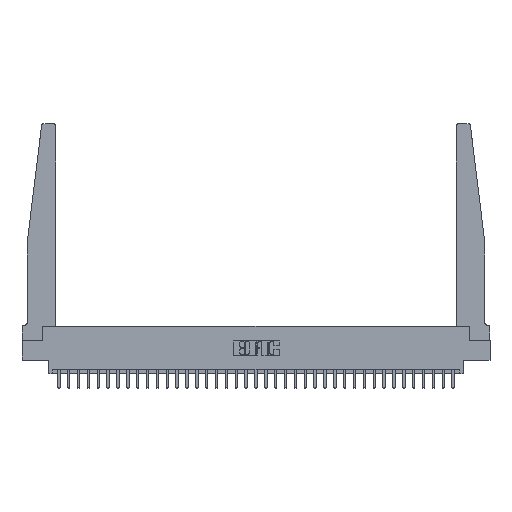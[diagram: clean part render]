
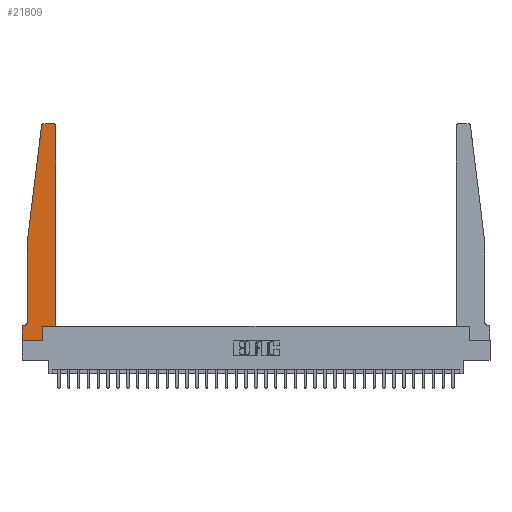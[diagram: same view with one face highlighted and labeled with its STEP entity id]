
A CAD part, top view. The second image highlights one B-rep face of the part: STEP entity #21809.
In plain terms, the highlighted planar face has unit normal (0, 0, 1).
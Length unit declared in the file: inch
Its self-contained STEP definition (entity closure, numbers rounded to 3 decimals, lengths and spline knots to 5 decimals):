
#943 = CARTESIAN_POINT ( 'NONE',  ( 0., 0., 0.37 ) ) ;
#962 = VERTEX_POINT ( 'NONE', #7965 ) ;
#1593 = CIRCLE ( 'NONE', #13711, 0.03 ) ;
#1871 = AXIS2_PLACEMENT_3D ( 'NONE', #12063, #29460, #30108 ) ;
#1919 = VECTOR ( 'NONE', #22863, 39.37008 ) ;
#2010 = CARTESIAN_POINT ( 'NONE',  ( 0.425, 0.18, 0.37 ) ) ;
#2086 = CARTESIAN_POINT ( 'NONE',  ( 0.065, 1.25, 0.37 ) ) ;
#2174 = DIRECTION ( 'NONE',  ( 0., 0., 1. ) ) ;
#2515 = CARTESIAN_POINT ( 'NONE',  ( 0., 0., 0.37 ) ) ;
#2569 = LINE ( 'NONE', #2086, #29321 ) ;
#2883 = CARTESIAN_POINT ( 'NONE',  ( 0.27653, 2.75, 0.37 ) ) ;
#3471 = CARTESIAN_POINT ( 'NONE',  ( 0.425, 0.18, 0.37 ) ) ;
#3569 = VERTEX_POINT ( 'NONE', #27847 ) ;
#3655 = CARTESIAN_POINT ( 'NONE',  ( 0.065, 0.1875, 0.37 ) ) ;
#4301 = ORIENTED_EDGE ( 'NONE', *, *, #28901, .T. ) ;
#5416 = ORIENTED_EDGE ( 'NONE', *, *, #29785, .T. ) ;
#5921 = CIRCLE ( 'NONE', #12198, 0.03 ) ;
#6221 = VECTOR ( 'NONE', #16796, 39.37008 ) ;
#6303 = EDGE_CURVE ( 'NONE', #18029, #8403, #32138, .T. ) ;
#6345 = ORIENTED_EDGE ( 'NONE', *, *, #8259, .T. ) ;
#6392 = VERTEX_POINT ( 'NONE', #14116 ) ;
#6654 = ORIENTED_EDGE ( 'NONE', *, *, #11583, .T. ) ;
#6799 = CARTESIAN_POINT ( 'NONE',  ( 0.25, 2.75, 0.37 ) ) ;
#7400 = ORIENTED_EDGE ( 'NONE', *, *, #25180, .T. ) ;
#7965 = CARTESIAN_POINT ( 'NONE',  ( 0.065, 1.25, 0.37 ) ) ;
#7969 = EDGE_CURVE ( 'NONE', #3569, #21873, #12035, .T. ) ;
#8115 = VERTEX_POINT ( 'NONE', #21014 ) ;
#8259 = EDGE_CURVE ( 'NONE', #16986, #6392, #22028, .T. ) ;
#8403 = VERTEX_POINT ( 'NONE', #2010 ) ;
#8548 = DIRECTION ( 'NONE',  ( 0., -1., 0. ) ) ;
#9052 = DIRECTION ( 'NONE',  ( 0., 0., -1. ) ) ;
#9510 = DIRECTION ( 'NONE',  ( 1., 0., 0. ) ) ;
#10059 = VECTOR ( 'NONE', #13225, 39.37008 ) ;
#10998 = DIRECTION ( 'NONE',  ( 0., 1., 0. ) ) ;
#11488 = CARTESIAN_POINT ( 'NONE',  ( 0., 0., 0.37 ) ) ;
#11583 = EDGE_CURVE ( 'NONE', #22275, #18432, #28152, .T. ) ;
#12035 = LINE ( 'NONE', #6799, #6221 ) ;
#12063 = CARTESIAN_POINT ( 'NONE',  ( 0., 0.1875, 0.37 ) ) ;
#12198 = AXIS2_PLACEMENT_3D ( 'NONE', #18623, #21079, #13717 ) ;
#12219 = CARTESIAN_POINT ( 'NONE',  ( 0.425, 2.72, 0.37 ) ) ;
#12319 = CARTESIAN_POINT ( 'NONE',  ( 0.395, 2.72, 0.37 ) ) ;
#13225 = DIRECTION ( 'NONE',  ( 1., 0., 0. ) ) ;
#13678 = EDGE_CURVE ( 'NONE', #27486, #962, #17900, .T. ) ;
#13711 = AXIS2_PLACEMENT_3D ( 'NONE', #12319, #2174, #17070 ) ;
#13717 = DIRECTION ( 'NONE',  ( 1., 0., 0. ) ) ;
#14116 = CARTESIAN_POINT ( 'NONE',  ( 0.015, 0.1875, 0.37 ) ) ;
#14307 = DIRECTION ( 'NONE',  ( -1., 0., 0. ) ) ;
#14493 = ORIENTED_EDGE ( 'NONE', *, *, #13678, .T. ) ;
#15130 = DIRECTION ( 'NONE',  ( -0.122, -0.992, 0. ) ) ;
#15173 = FACE_OUTER_BOUND ( 'NONE', #15773, .T. ) ;
#15477 = ORIENTED_EDGE ( 'NONE', *, *, #23230, .T. ) ;
#15773 = EDGE_LOOP ( 'NONE', ( #28804, #21388, #14493, #4301, #6345, #7400, #28339, #6654, #15477, #23433, #24573, #5416 ) ) ;
#15919 = LINE ( 'NONE', #3471, #27981 ) ;
#16796 = DIRECTION ( 'NONE',  ( -1., 0., 0. ) ) ;
#16986 = VERTEX_POINT ( 'NONE', #21519 ) ;
#17070 = DIRECTION ( 'NONE',  ( 1., 0., 0. ) ) ;
#17461 = PLANE ( 'NONE',  #1871 ) ;
#17900 = LINE ( 'NONE', #22816, #29016 ) ;
#18029 = VERTEX_POINT ( 'NONE', #22697 ) ;
#18432 = VERTEX_POINT ( 'NONE', #22808 ) ;
#18623 = CARTESIAN_POINT ( 'NONE',  ( 0.27653, 2.72, 0.37 ) ) ;
#19140 = EDGE_CURVE ( 'NONE', #21873, #27486, #5921, .T. ) ;
#19248 = VERTEX_POINT ( 'NONE', #12219 ) ;
#19409 = AXIS2_PLACEMENT_3D ( 'NONE', #26441, #9052, #14307 ) ;
#20860 = EDGE_CURVE ( 'NONE', #8403, #19248, #15919, .T. ) ;
#21014 = CARTESIAN_POINT ( 'NONE',  ( 0., 0.1875, 0.37 ) ) ;
#21079 = DIRECTION ( 'NONE',  ( 0., 0., 1. ) ) ;
#21388 = ORIENTED_EDGE ( 'NONE', *, *, #19140, .T. ) ;
#21519 = CARTESIAN_POINT ( 'NONE',  ( 0.065, 0.2375, 0.37 ) ) ;
#21809 = ADVANCED_FACE ( 'NONE', ( #15173 ), #17461, .T. ) ;
#21873 = VERTEX_POINT ( 'NONE', #2883 ) ;
#22028 = CIRCLE ( 'NONE', #19409, 0.05 ) ;
#22275 = VERTEX_POINT ( 'NONE', #2515 ) ;
#22387 = DIRECTION ( 'NONE',  ( 0., -1., 0. ) ) ;
#22697 = CARTESIAN_POINT ( 'NONE',  ( 0.2605, 0.18, 0.37 ) ) ;
#22808 = CARTESIAN_POINT ( 'NONE',  ( 0.2605, 0., 0.37 ) ) ;
#22816 = CARTESIAN_POINT ( 'NONE',  ( 0.065, 1.25, 0.37 ) ) ;
#22863 = DIRECTION ( 'NONE',  ( 0., 1., 0. ) ) ;
#23230 = EDGE_CURVE ( 'NONE', #18432, #18029, #27801, .T. ) ;
#23433 = ORIENTED_EDGE ( 'NONE', *, *, #6303, .T. ) ;
#23952 = LINE ( 'NONE', #11488, #24967 ) ;
#23989 = EDGE_CURVE ( 'NONE', #8115, #22275, #23952, .T. ) ;
#24573 = ORIENTED_EDGE ( 'NONE', *, *, #20860, .T. ) ;
#24967 = VECTOR ( 'NONE', #8548, 39.37008 ) ;
#25180 = EDGE_CURVE ( 'NONE', #6392, #8115, #31198, .T. ) ;
#26441 = CARTESIAN_POINT ( 'NONE',  ( 0.015, 0.2375, 0.37 ) ) ;
#27015 = CARTESIAN_POINT ( 'NONE',  ( 0.24675, 2.72367, 0.37 ) ) ;
#27486 = VERTEX_POINT ( 'NONE', #27015 ) ;
#27801 = LINE ( 'NONE', #27955, #1919 ) ;
#27847 = CARTESIAN_POINT ( 'NONE',  ( 0.395, 2.75, 0.37 ) ) ;
#27955 = CARTESIAN_POINT ( 'NONE',  ( 0.2605, 0.18, 0.37 ) ) ;
#27981 = VECTOR ( 'NONE', #10998, 39.37008 ) ;
#28152 = LINE ( 'NONE', #943, #10059 ) ;
#28339 = ORIENTED_EDGE ( 'NONE', *, *, #23989, .T. ) ;
#28804 = ORIENTED_EDGE ( 'NONE', *, *, #7969, .T. ) ;
#28901 = EDGE_CURVE ( 'NONE', #962, #16986, #2569, .T. ) ;
#28911 = DIRECTION ( 'NONE',  ( -1., 0., 0. ) ) ;
#29016 = VECTOR ( 'NONE', #15130, 39.37008 ) ;
#29109 = VECTOR ( 'NONE', #9510, 39.37008 ) ;
#29321 = VECTOR ( 'NONE', #22387, 39.37008 ) ;
#29460 = DIRECTION ( 'NONE',  ( 0., 0., 1. ) ) ;
#29785 = EDGE_CURVE ( 'NONE', #19248, #3569, #1593, .T. ) ;
#30108 = DIRECTION ( 'NONE',  ( 1., 0., 0. ) ) ;
#31198 = LINE ( 'NONE', #3655, #31439 ) ;
#31439 = VECTOR ( 'NONE', #28911, 39.37008 ) ;
#31506 = CARTESIAN_POINT ( 'NONE',  ( 0.425, 0.18, 0.37 ) ) ;
#32138 = LINE ( 'NONE', #31506, #29109 ) ;
